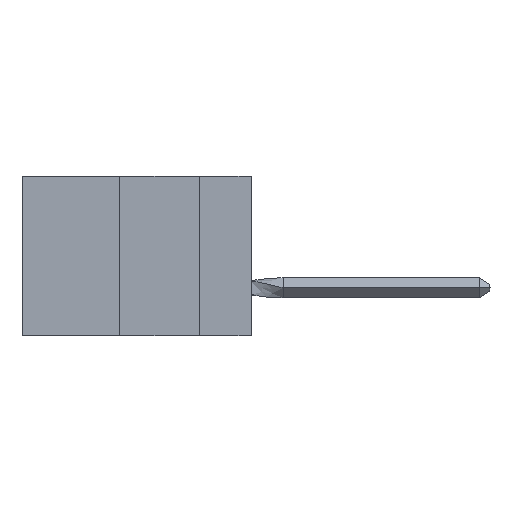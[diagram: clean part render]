
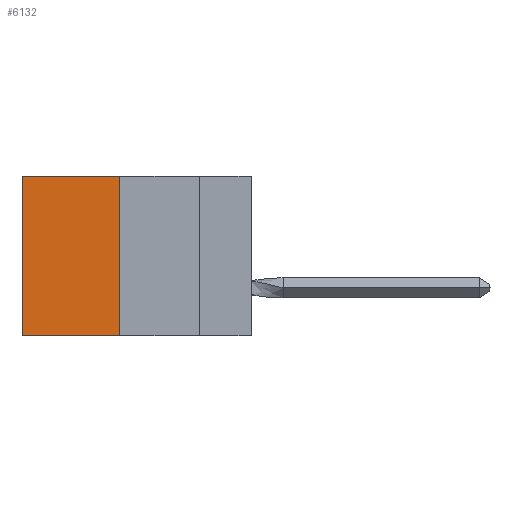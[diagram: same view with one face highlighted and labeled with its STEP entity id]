
A CAD part, left-side view. The second image highlights one B-rep face of the part: STEP entity #6132.
In plain terms, the highlighted planar face has unit normal (-1, 0, 0).
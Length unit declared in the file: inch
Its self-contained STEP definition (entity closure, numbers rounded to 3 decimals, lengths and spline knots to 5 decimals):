
#536 = ORIENTED_EDGE ( 'NONE', *, *, #6100, .F. ) ;
#1069 = CARTESIAN_POINT ( 'NONE',  ( 0.305, 0.413, -0.5 ) ) ;
#1252 = CARTESIAN_POINT ( 'NONE',  ( 0.305, 0.72, 0. ) ) ;
#1271 = EDGE_CURVE ( 'NONE', #6466, #2678, #3517, .T. ) ;
#1474 = ORIENTED_EDGE ( 'NONE', *, *, #4144, .T. ) ;
#1482 = VECTOR ( 'NONE', #9910, 39.37008 ) ;
#1738 = ORIENTED_EDGE ( 'NONE', *, *, #11596, .T. ) ;
#1818 = AXIS2_PLACEMENT_3D ( 'NONE', #1868, #7531, #6168 ) ;
#1868 = CARTESIAN_POINT ( 'NONE',  ( 0.305, 0.413, -0.5 ) ) ;
#2547 = CARTESIAN_POINT ( 'NONE',  ( 0.305, 0.413, 0. ) ) ;
#2580 = VERTEX_POINT ( 'NONE', #1252 ) ;
#2678 = VERTEX_POINT ( 'NONE', #6621 ) ;
#3517 = LINE ( 'NONE', #1069, #1482 ) ;
#3894 = DIRECTION ( 'NONE',  ( 0., 0., -1. ) ) ;
#4144 = EDGE_CURVE ( 'NONE', #6466, #2580, #8111, .T. ) ;
#4369 = LINE ( 'NONE', #12639, #10223 ) ;
#4640 = PLANE ( 'NONE',  #1818 ) ;
#6100 = EDGE_CURVE ( 'NONE', #2678, #16199, #13083, .T. ) ;
#6132 = ADVANCED_FACE ( 'NONE', ( #6727 ), #4640, .F. ) ;
#6168 = DIRECTION ( 'NONE',  ( 0., 0., -1. ) ) ;
#6466 = VERTEX_POINT ( 'NONE', #18640 ) ;
#6621 = CARTESIAN_POINT ( 'NONE',  ( 0.305, 0.413, -0.5 ) ) ;
#6727 = FACE_OUTER_BOUND ( 'NONE', #17560, .T. ) ;
#6884 = CARTESIAN_POINT ( 'NONE',  ( 0.305, 0.72, -0.5 ) ) ;
#7184 = VECTOR ( 'NONE', #14850, 39.37008 ) ;
#7531 = DIRECTION ( 'NONE',  ( 1., 0., 0. ) ) ;
#8111 = LINE ( 'NONE', #2547, #10376 ) ;
#9910 = DIRECTION ( 'NONE',  ( 0., 0., -1. ) ) ;
#10223 = VECTOR ( 'NONE', #3894, 39.37008 ) ;
#10376 = VECTOR ( 'NONE', #12677, 39.37008 ) ;
#11596 = EDGE_CURVE ( 'NONE', #2580, #16199, #4369, .T. ) ;
#11931 = CARTESIAN_POINT ( 'NONE',  ( 0.305, 0.413, -0.5 ) ) ;
#12639 = CARTESIAN_POINT ( 'NONE',  ( 0.305, 0.72, -0.5 ) ) ;
#12677 = DIRECTION ( 'NONE',  ( 0., 1., 0. ) ) ;
#13083 = LINE ( 'NONE', #11931, #7184 ) ;
#14850 = DIRECTION ( 'NONE',  ( 0., 1., 0. ) ) ;
#16199 = VERTEX_POINT ( 'NONE', #6884 ) ;
#16796 = ORIENTED_EDGE ( 'NONE', *, *, #1271, .F. ) ;
#17560 = EDGE_LOOP ( 'NONE', ( #1738, #536, #16796, #1474 ) ) ;
#18640 = CARTESIAN_POINT ( 'NONE',  ( 0.305, 0.413, 0. ) ) ;
